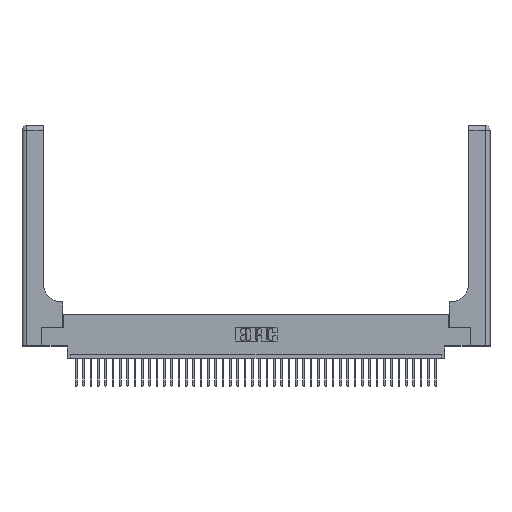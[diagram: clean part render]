
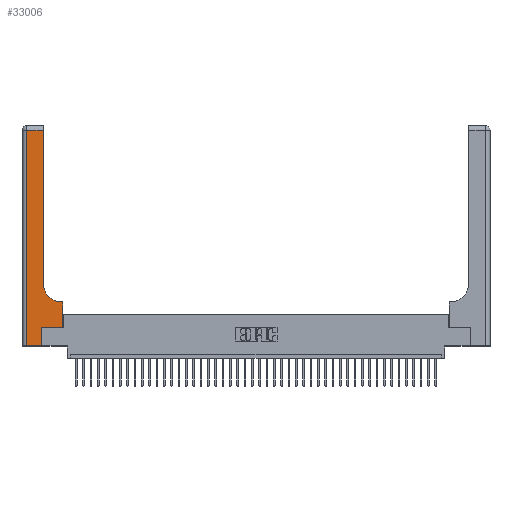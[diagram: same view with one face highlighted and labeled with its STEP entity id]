
A CAD part, top view. The second image highlights one B-rep face of the part: STEP entity #33006.
In plain terms, the highlighted planar face has unit normal (0, 0, 1).
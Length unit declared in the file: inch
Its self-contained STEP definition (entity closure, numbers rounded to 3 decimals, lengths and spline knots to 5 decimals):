
#492 = EDGE_CURVE ( 'NONE', #39546, #31968, #6762, .T. ) ;
#543 = VECTOR ( 'NONE', #17492, 39.37008 ) ;
#611 = ORIENTED_EDGE ( 'NONE', *, *, #1437, .T. ) ;
#1437 = EDGE_CURVE ( 'NONE', #2318, #39546, #9748, .T. ) ;
#1813 = AXIS2_PLACEMENT_3D ( 'NONE', #8550, #24804, #11845 ) ;
#2318 = VERTEX_POINT ( 'NONE', #20957 ) ;
#2571 = CARTESIAN_POINT ( 'NONE',  ( 0.2915, 3., 0.37 ) ) ;
#3465 = CARTESIAN_POINT ( 'NONE',  ( 0.269, 0.25, 0.37 ) ) ;
#5240 = AXIS2_PLACEMENT_3D ( 'NONE', #10310, #13426, #16426 ) ;
#5452 = CARTESIAN_POINT ( 'NONE',  ( 0.06, 3., 0.37 ) ) ;
#5685 = CIRCLE ( 'NONE', #1813, 0.25 ) ;
#6725 = VECTOR ( 'NONE', #18683, 39.37008 ) ;
#6762 = LINE ( 'NONE', #17661, #7758 ) ;
#7434 = CARTESIAN_POINT ( 'NONE',  ( 0., 0., 0.37 ) ) ;
#7758 = VECTOR ( 'NONE', #22537, 39.37008 ) ;
#8261 = CARTESIAN_POINT ( 'NONE',  ( 0.2915, 2.94, 0.37 ) ) ;
#8519 = ORIENTED_EDGE ( 'NONE', *, *, #35103, .T. ) ;
#8550 = CARTESIAN_POINT ( 'NONE',  ( 0.5415, 0.85, 0.37 ) ) ;
#9052 = CARTESIAN_POINT ( 'NONE',  ( 0.269, 0., 0.37 ) ) ;
#9437 = VERTEX_POINT ( 'NONE', #34161 ) ;
#9748 = LINE ( 'NONE', #3465, #543 ) ;
#10310 = CARTESIAN_POINT ( 'NONE',  ( 0., 3., 0.37 ) ) ;
#11845 = DIRECTION ( 'NONE',  ( 1., 0., 0. ) ) ;
#12049 = CARTESIAN_POINT ( 'NONE',  ( 0.2915, 0.6, 0.37 ) ) ;
#12161 = EDGE_CURVE ( 'NONE', #31968, #9437, #23442, .T. ) ;
#12237 = VECTOR ( 'NONE', #15778, 39.37008 ) ;
#13193 = LINE ( 'NONE', #41863, #12237 ) ;
#13289 = PLANE ( 'NONE',  #5240 ) ;
#13426 = DIRECTION ( 'NONE',  ( 0., 0., -1. ) ) ;
#13894 = VECTOR ( 'NONE', #30867, 39.37008 ) ;
#14311 = LINE ( 'NONE', #40961, #6725 ) ;
#15778 = DIRECTION ( 'NONE',  ( -1., 0., 0. ) ) ;
#16426 = DIRECTION ( 'NONE',  ( -1., 0., 0. ) ) ;
#17492 = DIRECTION ( 'NONE',  ( 1., 0., 0. ) ) ;
#17553 = EDGE_CURVE ( 'NONE', #34115, #34479, #13193, .T. ) ;
#17661 = CARTESIAN_POINT ( 'NONE',  ( 0.5585, 0.25, 0.37 ) ) ;
#18683 = DIRECTION ( 'NONE',  ( 0., 1., 0. ) ) ;
#19803 = LINE ( 'NONE', #2571, #24289 ) ;
#20007 = CARTESIAN_POINT ( 'NONE',  ( 0.5585, 0.25, 0.37 ) ) ;
#20957 = CARTESIAN_POINT ( 'NONE',  ( 0.269, 0.25, 0.37 ) ) ;
#21055 = EDGE_CURVE ( 'NONE', #38438, #34115, #19803, .T. ) ;
#21509 = LINE ( 'NONE', #5452, #13894 ) ;
#21666 = DIRECTION ( 'NONE',  ( 0., 1., 0. ) ) ;
#22537 = DIRECTION ( 'NONE',  ( 0., 1., 0. ) ) ;
#23402 = DIRECTION ( 'NONE',  ( 1., 0., 0. ) ) ;
#23442 = LINE ( 'NONE', #12049, #29541 ) ;
#24289 = VECTOR ( 'NONE', #21666, 39.37008 ) ;
#24534 = VERTEX_POINT ( 'NONE', #9052 ) ;
#24804 = DIRECTION ( 'NONE',  ( 0., 0., -1. ) ) ;
#25293 = VECTOR ( 'NONE', #23402, 39.37008 ) ;
#25387 = ORIENTED_EDGE ( 'NONE', *, *, #21055, .T. ) ;
#26628 = EDGE_CURVE ( 'NONE', #9437, #38438, #5685, .T. ) ;
#26751 = ORIENTED_EDGE ( 'NONE', *, *, #27843, .T. ) ;
#27396 = FACE_OUTER_BOUND ( 'NONE', #32953, .T. ) ;
#27843 = EDGE_CURVE ( 'NONE', #32797, #24534, #36327, .T. ) ;
#28202 = CARTESIAN_POINT ( 'NONE',  ( 0.06, 0., 0.37 ) ) ;
#28340 = ORIENTED_EDGE ( 'NONE', *, *, #34092, .T. ) ;
#29541 = VECTOR ( 'NONE', #30807, 39.37008 ) ;
#30807 = DIRECTION ( 'NONE',  ( -1., 0., 0. ) ) ;
#30867 = DIRECTION ( 'NONE',  ( 0., -1., 0. ) ) ;
#31144 = ORIENTED_EDGE ( 'NONE', *, *, #12161, .T. ) ;
#31968 = VERTEX_POINT ( 'NONE', #33362 ) ;
#32797 = VERTEX_POINT ( 'NONE', #28202 ) ;
#32953 = EDGE_LOOP ( 'NONE', ( #25387, #41342, #28340, #26751, #8519, #611, #38848, #31144, #37635 ) ) ;
#33006 = ADVANCED_FACE ( 'NONE', ( #27396 ), #13289, .F. ) ;
#33362 = CARTESIAN_POINT ( 'NONE',  ( 0.5585, 0.6, 0.37 ) ) ;
#34092 = EDGE_CURVE ( 'NONE', #34479, #32797, #21509, .T. ) ;
#34115 = VERTEX_POINT ( 'NONE', #8261 ) ;
#34161 = CARTESIAN_POINT ( 'NONE',  ( 0.5415, 0.6, 0.37 ) ) ;
#34479 = VERTEX_POINT ( 'NONE', #36403 ) ;
#35103 = EDGE_CURVE ( 'NONE', #24534, #2318, #14311, .T. ) ;
#36327 = LINE ( 'NONE', #7434, #25293 ) ;
#36403 = CARTESIAN_POINT ( 'NONE',  ( 0.06, 2.94, 0.37 ) ) ;
#37635 = ORIENTED_EDGE ( 'NONE', *, *, #26628, .T. ) ;
#38438 = VERTEX_POINT ( 'NONE', #39757 ) ;
#38848 = ORIENTED_EDGE ( 'NONE', *, *, #492, .T. ) ;
#39546 = VERTEX_POINT ( 'NONE', #20007 ) ;
#39757 = CARTESIAN_POINT ( 'NONE',  ( 0.2915, 0.85, 0.37 ) ) ;
#40961 = CARTESIAN_POINT ( 'NONE',  ( 0.269, 0., 0.37 ) ) ;
#41342 = ORIENTED_EDGE ( 'NONE', *, *, #17553, .T. ) ;
#41863 = CARTESIAN_POINT ( 'NONE',  ( 0., 2.94, 0.37 ) ) ;
